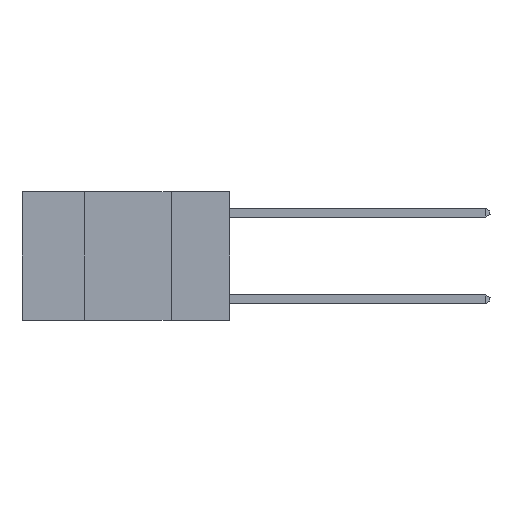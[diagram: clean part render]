
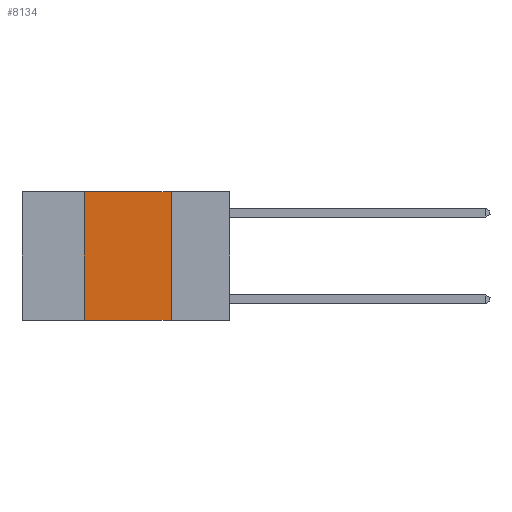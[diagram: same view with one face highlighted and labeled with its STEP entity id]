
A CAD part, left-side view. The second image highlights one B-rep face of the part: STEP entity #8134.
In plain terms, the highlighted planar face has unit normal (-1, 0, 0).
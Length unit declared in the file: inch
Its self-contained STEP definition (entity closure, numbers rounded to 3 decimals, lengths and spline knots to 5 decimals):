
#41 = PLANE ( 'NONE',  #1918 ) ;
#402 = VECTOR ( 'NONE', #10144, 39.37008 ) ;
#738 = ORIENTED_EDGE ( 'NONE', *, *, #4482, .T. ) ;
#1219 = EDGE_CURVE ( 'NONE', #8102, #2805, #7662, .T. ) ;
#1440 = CARTESIAN_POINT ( 'NONE',  ( 0., 0.42, 0. ) ) ;
#1554 = EDGE_CURVE ( 'NONE', #4982, #2570, #12293, .T. ) ;
#1737 = VECTOR ( 'NONE', #7079, 39.37008 ) ;
#1918 = AXIS2_PLACEMENT_3D ( 'NONE', #4996, #8770, #13798 ) ;
#2224 = CARTESIAN_POINT ( 'NONE',  ( 0., 0.6, 0. ) ) ;
#2570 = VERTEX_POINT ( 'NONE', #1440 ) ;
#2805 = VERTEX_POINT ( 'NONE', #8401 ) ;
#3084 = ORIENTED_EDGE ( 'NONE', *, *, #11078, .F. ) ;
#3240 = VECTOR ( 'NONE', #11471, 39.37008 ) ;
#3567 = VECTOR ( 'NONE', #12524, 39.37008 ) ;
#4482 = EDGE_CURVE ( 'NONE', #4982, #2805, #6774, .T. ) ;
#4982 = VERTEX_POINT ( 'NONE', #10793 ) ;
#4996 = CARTESIAN_POINT ( 'NONE',  ( 0., 0.6, 0. ) ) ;
#5866 = CARTESIAN_POINT ( 'NONE',  ( 0., 0.6, -0.37 ) ) ;
#6774 = LINE ( 'NONE', #5866, #1737 ) ;
#7079 = DIRECTION ( 'NONE',  ( 0., -1., 0. ) ) ;
#7561 = CARTESIAN_POINT ( 'NONE',  ( 0., 0.42, 0. ) ) ;
#7662 = LINE ( 'NONE', #13921, #3240 ) ;
#8102 = VERTEX_POINT ( 'NONE', #12677 ) ;
#8134 = ADVANCED_FACE ( 'NONE', ( #14933 ), #41, .F. ) ;
#8263 = ORIENTED_EDGE ( 'NONE', *, *, #1554, .F. ) ;
#8401 = CARTESIAN_POINT ( 'NONE',  ( 0., 0.17, -0.37 ) ) ;
#8451 = LINE ( 'NONE', #2224, #402 ) ;
#8770 = DIRECTION ( 'NONE',  ( 1., 0., 0. ) ) ;
#9894 = ORIENTED_EDGE ( 'NONE', *, *, #1219, .F. ) ;
#10144 = DIRECTION ( 'NONE',  ( 0., -1., 0. ) ) ;
#10793 = CARTESIAN_POINT ( 'NONE',  ( 0., 0.42, -0.37 ) ) ;
#11078 = EDGE_CURVE ( 'NONE', #2570, #8102, #8451, .T. ) ;
#11471 = DIRECTION ( 'NONE',  ( 0., 0., -1. ) ) ;
#11856 = EDGE_LOOP ( 'NONE', ( #9894, #3084, #8263, #738 ) ) ;
#12293 = LINE ( 'NONE', #7561, #3567 ) ;
#12524 = DIRECTION ( 'NONE',  ( 0., 0., 1. ) ) ;
#12677 = CARTESIAN_POINT ( 'NONE',  ( 0., 0.17, 0. ) ) ;
#13798 = DIRECTION ( 'NONE',  ( 0., 0., -1. ) ) ;
#13921 = CARTESIAN_POINT ( 'NONE',  ( 0., 0.17, 0. ) ) ;
#14933 = FACE_OUTER_BOUND ( 'NONE', #11856, .T. ) ;
